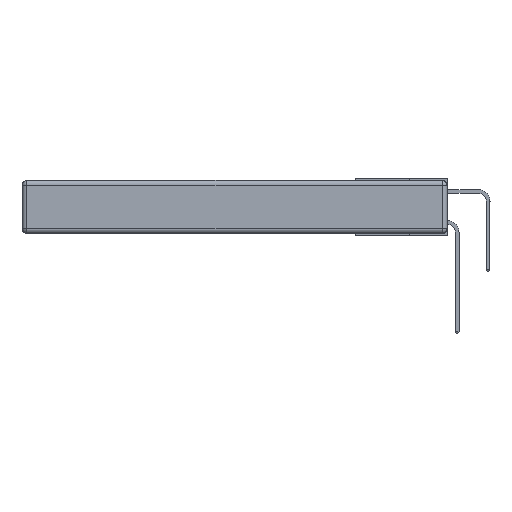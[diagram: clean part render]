
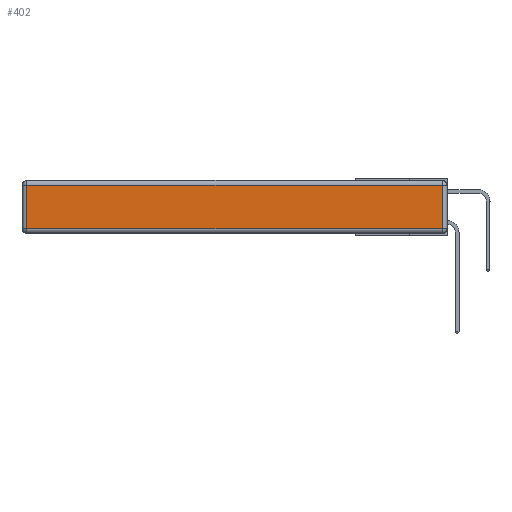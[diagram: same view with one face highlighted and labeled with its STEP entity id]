
A CAD part, left-side view. The second image highlights one B-rep face of the part: STEP entity #402.
In plain terms, the highlighted planar face has unit normal (-1, 0, 0).
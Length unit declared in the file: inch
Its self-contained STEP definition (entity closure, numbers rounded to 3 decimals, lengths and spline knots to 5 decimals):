
#402 = ADVANCED_FACE ( 'NONE', ( #9647 ), #22151, .T. ) ;
#646 = VERTEX_POINT ( 'NONE', #20280 ) ;
#1450 = LINE ( 'NONE', #13137, #9958 ) ;
#2189 = VECTOR ( 'NONE', #16501, 39.37008 ) ;
#2294 = EDGE_CURVE ( 'NONE', #646, #7069, #23267, .T. ) ;
#2608 = CARTESIAN_POINT ( 'NONE',  ( 0., 0.03, -0.03 ) ) ;
#3254 = LINE ( 'NONE', #4817, #17351 ) ;
#4817 = CARTESIAN_POINT ( 'NONE',  ( 0., 2.72, -0.343 ) ) ;
#5788 = VERTEX_POINT ( 'NONE', #2608 ) ;
#6131 = AXIS2_PLACEMENT_3D ( 'NONE', #11024, #20505, #11184 ) ;
#6848 = EDGE_CURVE ( 'NONE', #8129, #646, #3254, .T. ) ;
#7069 = VERTEX_POINT ( 'NONE', #7529 ) ;
#7529 = CARTESIAN_POINT ( 'NONE',  ( 0., 0.03, -0.313 ) ) ;
#8129 = VERTEX_POINT ( 'NONE', #19741 ) ;
#9639 = CARTESIAN_POINT ( 'NONE',  ( 0., 0.03, -0.343 ) ) ;
#9647 = FACE_OUTER_BOUND ( 'NONE', #10713, .T. ) ;
#9958 = VECTOR ( 'NONE', #13385, 39.37008 ) ;
#10043 = ORIENTED_EDGE ( 'NONE', *, *, #2294, .T. ) ;
#10713 = EDGE_LOOP ( 'NONE', ( #10043, #16633, #13732, #15247 ) ) ;
#11024 = CARTESIAN_POINT ( 'NONE',  ( 0., 0., -0.343 ) ) ;
#11184 = DIRECTION ( 'NONE',  ( 0., 0., 1. ) ) ;
#13137 = CARTESIAN_POINT ( 'NONE',  ( 0., 2.75, -0.03 ) ) ;
#13385 = DIRECTION ( 'NONE',  ( 0., 1., 0. ) ) ;
#13732 = ORIENTED_EDGE ( 'NONE', *, *, #16725, .T. ) ;
#14462 = CARTESIAN_POINT ( 'NONE',  ( 0., 0., -0.313 ) ) ;
#15011 = DIRECTION ( 'NONE',  ( 0., 0., 1. ) ) ;
#15247 = ORIENTED_EDGE ( 'NONE', *, *, #6848, .T. ) ;
#16103 = EDGE_CURVE ( 'NONE', #7069, #5788, #23430, .T. ) ;
#16501 = DIRECTION ( 'NONE',  ( 0., -1., 0. ) ) ;
#16633 = ORIENTED_EDGE ( 'NONE', *, *, #16103, .T. ) ;
#16725 = EDGE_CURVE ( 'NONE', #5788, #8129, #1450, .T. ) ;
#17351 = VECTOR ( 'NONE', #17630, 39.37008 ) ;
#17630 = DIRECTION ( 'NONE',  ( 0., 0., -1. ) ) ;
#19741 = CARTESIAN_POINT ( 'NONE',  ( 0., 2.72, -0.03 ) ) ;
#19947 = VECTOR ( 'NONE', #15011, 39.37008 ) ;
#20280 = CARTESIAN_POINT ( 'NONE',  ( 0., 2.72, -0.313 ) ) ;
#20505 = DIRECTION ( 'NONE',  ( -1., 0., 0. ) ) ;
#22151 = PLANE ( 'NONE',  #6131 ) ;
#23267 = LINE ( 'NONE', #14462, #2189 ) ;
#23430 = LINE ( 'NONE', #9639, #19947 ) ;
